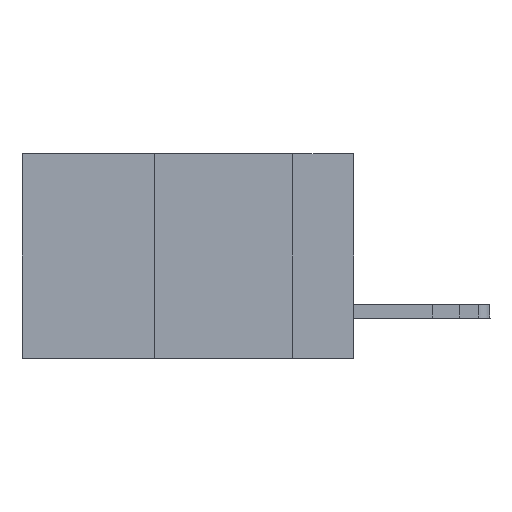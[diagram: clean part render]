
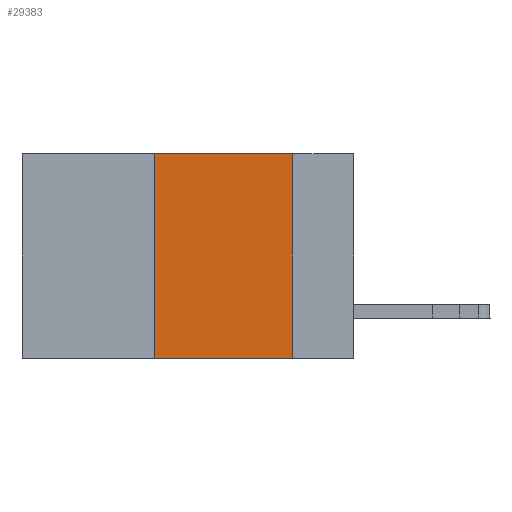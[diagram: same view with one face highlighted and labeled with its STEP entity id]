
A CAD part, left-side view. The second image highlights one B-rep face of the part: STEP entity #29383.
In plain terms, the highlighted planar face has unit normal (-1, 0, 0).
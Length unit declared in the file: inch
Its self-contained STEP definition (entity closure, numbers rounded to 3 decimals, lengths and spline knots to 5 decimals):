
#447 = CARTESIAN_POINT ( 'NONE',  ( 0., 0.6, 0. ) ) ;
#1065 = AXIS2_PLACEMENT_3D ( 'NONE', #447, #18710, #11907 ) ;
#3249 = EDGE_CURVE ( 'NONE', #3776, #21729, #31553, .T. ) ;
#3448 = DIRECTION ( 'NONE',  ( 0., 0., -1. ) ) ;
#3776 = VERTEX_POINT ( 'NONE', #7597 ) ;
#4814 = VECTOR ( 'NONE', #26154, 39.37008 ) ;
#6194 = EDGE_CURVE ( 'NONE', #3776, #22234, #22153, .T. ) ;
#7597 = CARTESIAN_POINT ( 'NONE',  ( 0., 0.36, -0.37 ) ) ;
#9267 = PLANE ( 'NONE',  #1065 ) ;
#10273 = CARTESIAN_POINT ( 'NONE',  ( 0., 0.6, -0.37 ) ) ;
#10490 = VECTOR ( 'NONE', #28365, 39.37008 ) ;
#11433 = EDGE_CURVE ( 'NONE', #21729, #35792, #12614, .T. ) ;
#11900 = ORIENTED_EDGE ( 'NONE', *, *, #3249, .F. ) ;
#11907 = DIRECTION ( 'NONE',  ( 0., 0., -1. ) ) ;
#12614 = LINE ( 'NONE', #39535, #28415 ) ;
#13626 = CARTESIAN_POINT ( 'NONE',  ( 0., 0.11, 0. ) ) ;
#15371 = ORIENTED_EDGE ( 'NONE', *, *, #6194, .T. ) ;
#16644 = LINE ( 'NONE', #13626, #35299 ) ;
#18710 = DIRECTION ( 'NONE',  ( 1., 0., 0. ) ) ;
#19159 = EDGE_CURVE ( 'NONE', #35792, #22234, #16644, .T. ) ;
#19971 = CARTESIAN_POINT ( 'NONE',  ( 0., 0.11, 0. ) ) ;
#21729 = VERTEX_POINT ( 'NONE', #31430 ) ;
#22153 = LINE ( 'NONE', #10273, #10490 ) ;
#22234 = VERTEX_POINT ( 'NONE', #35786 ) ;
#26154 = DIRECTION ( 'NONE',  ( 0., 0., 1. ) ) ;
#28365 = DIRECTION ( 'NONE',  ( 0., -1., 0. ) ) ;
#28415 = VECTOR ( 'NONE', #30517, 39.37008 ) ;
#29383 = ADVANCED_FACE ( 'NONE', ( #36785 ), #9267, .F. ) ;
#29494 = EDGE_LOOP ( 'NONE', ( #34865, #34653, #11900, #15371 ) ) ;
#30517 = DIRECTION ( 'NONE',  ( 0., -1., 0. ) ) ;
#31430 = CARTESIAN_POINT ( 'NONE',  ( 0., 0.36, 0. ) ) ;
#31553 = LINE ( 'NONE', #31965, #4814 ) ;
#31965 = CARTESIAN_POINT ( 'NONE',  ( 0., 0.36, 0. ) ) ;
#34653 = ORIENTED_EDGE ( 'NONE', *, *, #11433, .F. ) ;
#34865 = ORIENTED_EDGE ( 'NONE', *, *, #19159, .F. ) ;
#35299 = VECTOR ( 'NONE', #3448, 39.37008 ) ;
#35786 = CARTESIAN_POINT ( 'NONE',  ( 0., 0.11, -0.37 ) ) ;
#35792 = VERTEX_POINT ( 'NONE', #19971 ) ;
#36785 = FACE_OUTER_BOUND ( 'NONE', #29494, .T. ) ;
#39535 = CARTESIAN_POINT ( 'NONE',  ( 0., 0.6, 0. ) ) ;
